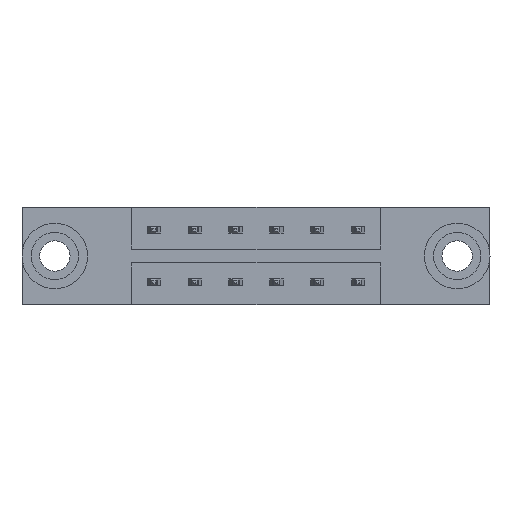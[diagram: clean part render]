
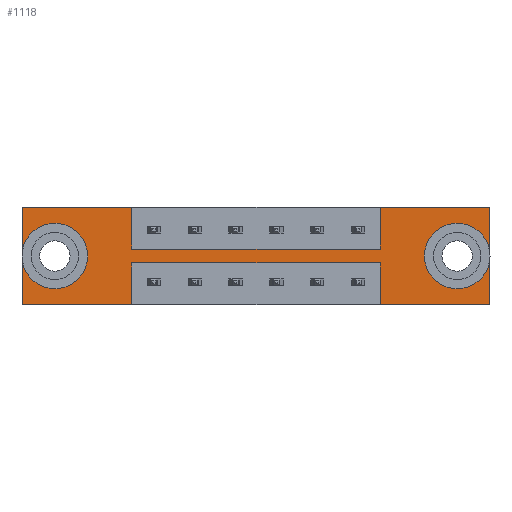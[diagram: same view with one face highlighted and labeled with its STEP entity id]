
A CAD part, front view. The second image highlights one B-rep face of the part: STEP entity #1118.
In plain terms, the highlighted planar face has unit normal (0, -1, 0).
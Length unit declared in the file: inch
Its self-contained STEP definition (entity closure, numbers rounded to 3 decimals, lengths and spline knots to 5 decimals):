
#32 = DIRECTION ( 'NONE',  ( 1., 0., 0. ) ) ;
#90 = VECTOR ( 'NONE', #867, 39.37008 ) ;
#153 = ORIENTED_EDGE ( 'NONE', *, *, #6819, .F. ) ;
#166 = CARTESIAN_POINT ( 'NONE',  ( 0., 0., 0. ) ) ;
#227 = DIRECTION ( 'NONE',  ( 0., 0., 1. ) ) ;
#283 = VERTEX_POINT ( 'NONE', #3975 ) ;
#312 = VERTEX_POINT ( 'NONE', #690 ) ;
#335 = EDGE_CURVE ( 'NONE', #312, #6142, #4841, .T. ) ;
#435 = LINE ( 'NONE', #8490, #8972 ) ;
#445 = DIRECTION ( 'NONE',  ( 0., 0., -1. ) ) ;
#528 = CARTESIAN_POINT ( 'NONE',  ( 0.4175, 0., -0.1585 ) ) ;
#538 = DIRECTION ( 'NONE',  ( 0., 0., -1. ) ) ;
#555 = EDGE_LOOP ( 'NONE', ( #7140, #1626 ) ) ;
#556 = EDGE_CURVE ( 'NONE', #1674, #4452, #4484, .T. ) ;
#621 = ORIENTED_EDGE ( 'NONE', *, *, #6482, .F. ) ;
#690 = CARTESIAN_POINT ( 'NONE',  ( 0.125, 0., -0.263 ) ) ;
#728 = CARTESIAN_POINT ( 'NONE',  ( 1.3665, 0., -0.1585 ) ) ;
#773 = CARTESIAN_POINT ( 'NONE',  ( 1.784, 0., 0. ) ) ;
#844 = ORIENTED_EDGE ( 'NONE', *, *, #7624, .F. ) ;
#867 = DIRECTION ( 'NONE',  ( 0., 0., 1. ) ) ;
#1046 = LINE ( 'NONE', #9149, #8395 ) ;
#1118 = ADVANCED_FACE ( 'NONE', ( #2104, #5496, #7355 ), #1302, .T. ) ;
#1302 = PLANE ( 'NONE',  #3380 ) ;
#1351 = VERTEX_POINT ( 'NONE', #7429 ) ;
#1425 = CARTESIAN_POINT ( 'NONE',  ( 0., 0., -0.37 ) ) ;
#1592 = LINE ( 'NONE', #8271, #6138 ) ;
#1626 = ORIENTED_EDGE ( 'NONE', *, *, #7099, .T. ) ;
#1674 = VERTEX_POINT ( 'NONE', #3363 ) ;
#1823 = CARTESIAN_POINT ( 'NONE',  ( 0.4175, 0., -0.1585 ) ) ;
#1852 = ORIENTED_EDGE ( 'NONE', *, *, #8261, .F. ) ;
#1972 = VERTEX_POINT ( 'NONE', #3911 ) ;
#2020 = DIRECTION ( 'NONE',  ( 0., 0., -1. ) ) ;
#2021 = VERTEX_POINT ( 'NONE', #8206 ) ;
#2055 = DIRECTION ( 'NONE',  ( -1., 0., 0. ) ) ;
#2104 = FACE_BOUND ( 'NONE', #555, .T. ) ;
#2151 = CARTESIAN_POINT ( 'NONE',  ( 0., 0., -0.37 ) ) ;
#2260 = DIRECTION ( 'NONE',  ( 0., -1., 0. ) ) ;
#2391 = EDGE_CURVE ( 'NONE', #6142, #312, #8800, .T. ) ;
#2453 = LINE ( 'NONE', #528, #6045 ) ;
#2458 = VERTEX_POINT ( 'NONE', #1425 ) ;
#2579 = ORIENTED_EDGE ( 'NONE', *, *, #3191, .F. ) ;
#2624 = VECTOR ( 'NONE', #5005, 39.37008 ) ;
#2634 = CARTESIAN_POINT ( 'NONE',  ( 1.659, 0., -0.263 ) ) ;
#2798 = CARTESIAN_POINT ( 'NONE',  ( 1.784, 0., -0.37 ) ) ;
#3191 = EDGE_CURVE ( 'NONE', #2458, #3700, #5799, .T. ) ;
#3336 = EDGE_CURVE ( 'NONE', #5399, #4900, #6786, .T. ) ;
#3363 = CARTESIAN_POINT ( 'NONE',  ( 1.3665, 0., 0. ) ) ;
#3380 = AXIS2_PLACEMENT_3D ( 'NONE', #2151, #2260, #2020 ) ;
#3385 = CARTESIAN_POINT ( 'NONE',  ( 0.125, 0., -0.185 ) ) ;
#3482 = EDGE_LOOP ( 'NONE', ( #1852, #7568, #153, #4021, #5942, #7802, #8017, #621, #2579, #4474, #8227, #844 ) ) ;
#3700 = VERTEX_POINT ( 'NONE', #8717 ) ;
#3808 = EDGE_CURVE ( 'NONE', #7415, #7008, #6336, .T. ) ;
#3911 = CARTESIAN_POINT ( 'NONE',  ( 0.4175, 0., -0.37 ) ) ;
#3951 = LINE ( 'NONE', #7084, #7502 ) ;
#3975 = CARTESIAN_POINT ( 'NONE',  ( 1.3665, 0., -0.2115 ) ) ;
#4021 = ORIENTED_EDGE ( 'NONE', *, *, #556, .F. ) ;
#4245 = DIRECTION ( 'NONE',  ( 0., 0., -1. ) ) ;
#4259 = DIRECTION ( 'NONE',  ( 0., 1., 0. ) ) ;
#4308 = CARTESIAN_POINT ( 'NONE',  ( 1.659, 0., -0.185 ) ) ;
#4431 = VECTOR ( 'NONE', #8244, 39.37008 ) ;
#4435 = VECTOR ( 'NONE', #445, 39.37008 ) ;
#4452 = VERTEX_POINT ( 'NONE', #5290 ) ;
#4474 = ORIENTED_EDGE ( 'NONE', *, *, #5937, .F. ) ;
#4482 = EDGE_CURVE ( 'NONE', #6966, #8374, #6436, .T. ) ;
#4484 = LINE ( 'NONE', #166, #4719 ) ;
#4719 = VECTOR ( 'NONE', #32, 39.37008 ) ;
#4841 = CIRCLE ( 'NONE', #4905, 0.078 ) ;
#4900 = VERTEX_POINT ( 'NONE', #2634 ) ;
#4905 = AXIS2_PLACEMENT_3D ( 'NONE', #3385, #5890, #6672 ) ;
#5005 = DIRECTION ( 'NONE',  ( -1., 0., 0. ) ) ;
#5064 = CARTESIAN_POINT ( 'NONE',  ( 0., 0., -0.37 ) ) ;
#5273 = EDGE_CURVE ( 'NONE', #1351, #7415, #2453, .T. ) ;
#5290 = CARTESIAN_POINT ( 'NONE',  ( 1.784, 0., 0. ) ) ;
#5399 = VERTEX_POINT ( 'NONE', #7959 ) ;
#5494 = ORIENTED_EDGE ( 'NONE', *, *, #2391, .T. ) ;
#5496 = FACE_BOUND ( 'NONE', #6860, .T. ) ;
#5787 = CIRCLE ( 'NONE', #8118, 0.078 ) ;
#5799 = LINE ( 'NONE', #6702, #9199 ) ;
#5887 = LINE ( 'NONE', #5931, #90 ) ;
#5890 = DIRECTION ( 'NONE',  ( 0., 1., 0. ) ) ;
#5931 = CARTESIAN_POINT ( 'NONE',  ( 1.3665, 0., -0.1585 ) ) ;
#5937 = EDGE_CURVE ( 'NONE', #1972, #2458, #1046, .T. ) ;
#5942 = ORIENTED_EDGE ( 'NONE', *, *, #7806, .F. ) ;
#6045 = VECTOR ( 'NONE', #538, 39.37008 ) ;
#6138 = VECTOR ( 'NONE', #8538, 39.37008 ) ;
#6142 = VERTEX_POINT ( 'NONE', #6556 ) ;
#6336 = LINE ( 'NONE', #8282, #4431 ) ;
#6343 = LINE ( 'NONE', #773, #4435 ) ;
#6362 = DIRECTION ( 'NONE',  ( 0., 0., 1. ) ) ;
#6436 = LINE ( 'NONE', #5064, #2624 ) ;
#6467 = AXIS2_PLACEMENT_3D ( 'NONE', #4308, #4259, #4245 ) ;
#6482 = EDGE_CURVE ( 'NONE', #3700, #1351, #1592, .T. ) ;
#6525 = AXIS2_PLACEMENT_3D ( 'NONE', #7811, #8815, #227 ) ;
#6556 = CARTESIAN_POINT ( 'NONE',  ( 0.125, 0., -0.107 ) ) ;
#6672 = DIRECTION ( 'NONE',  ( 0., 0., 1. ) ) ;
#6702 = CARTESIAN_POINT ( 'NONE',  ( 0., 0., 0. ) ) ;
#6786 = CIRCLE ( 'NONE', #6467, 0.078 ) ;
#6819 = EDGE_CURVE ( 'NONE', #4452, #6966, #6343, .T. ) ;
#6860 = EDGE_LOOP ( 'NONE', ( #5494, #7354 ) ) ;
#6966 = VERTEX_POINT ( 'NONE', #2798 ) ;
#6984 = VECTOR ( 'NONE', #7485, 39.37008 ) ;
#7008 = VERTEX_POINT ( 'NONE', #728 ) ;
#7084 = CARTESIAN_POINT ( 'NONE',  ( 1.3665, 0., -0.2115 ) ) ;
#7099 = EDGE_CURVE ( 'NONE', #4900, #5399, #5787, .T. ) ;
#7140 = ORIENTED_EDGE ( 'NONE', *, *, #3336, .T. ) ;
#7163 = EDGE_CURVE ( 'NONE', #2021, #1972, #9189, .T. ) ;
#7232 = CARTESIAN_POINT ( 'NONE',  ( 1.3665, 0., -0.37 ) ) ;
#7354 = ORIENTED_EDGE ( 'NONE', *, *, #335, .T. ) ;
#7355 = FACE_OUTER_BOUND ( 'NONE', #3482, .T. ) ;
#7386 = CARTESIAN_POINT ( 'NONE',  ( 0.4175, 0., -0.2115 ) ) ;
#7415 = VERTEX_POINT ( 'NONE', #1823 ) ;
#7429 = CARTESIAN_POINT ( 'NONE',  ( 0.4175, 0., 0. ) ) ;
#7485 = DIRECTION ( 'NONE',  ( 0., 0., -1. ) ) ;
#7502 = VECTOR ( 'NONE', #7787, 39.37008 ) ;
#7568 = ORIENTED_EDGE ( 'NONE', *, *, #4482, .F. ) ;
#7624 = EDGE_CURVE ( 'NONE', #283, #2021, #435, .T. ) ;
#7787 = DIRECTION ( 'NONE',  ( 0., 0., 1. ) ) ;
#7802 = ORIENTED_EDGE ( 'NONE', *, *, #3808, .F. ) ;
#7806 = EDGE_CURVE ( 'NONE', #7008, #1674, #5887, .T. ) ;
#7811 = CARTESIAN_POINT ( 'NONE',  ( 0.125, 0., -0.185 ) ) ;
#7831 = DIRECTION ( 'NONE',  ( -1., 0., 0. ) ) ;
#7959 = CARTESIAN_POINT ( 'NONE',  ( 1.659, 0., -0.107 ) ) ;
#7995 = DIRECTION ( 'NONE',  ( 0., 0., -1. ) ) ;
#8017 = ORIENTED_EDGE ( 'NONE', *, *, #5273, .F. ) ;
#8022 = DIRECTION ( 'NONE',  ( 0., 1., 0. ) ) ;
#8048 = CARTESIAN_POINT ( 'NONE',  ( 1.659, 0., -0.185 ) ) ;
#8118 = AXIS2_PLACEMENT_3D ( 'NONE', #8048, #8022, #7995 ) ;
#8206 = CARTESIAN_POINT ( 'NONE',  ( 0.4175, 0., -0.2115 ) ) ;
#8227 = ORIENTED_EDGE ( 'NONE', *, *, #7163, .F. ) ;
#8244 = DIRECTION ( 'NONE',  ( 1., 0., 0. ) ) ;
#8261 = EDGE_CURVE ( 'NONE', #8374, #283, #3951, .T. ) ;
#8271 = CARTESIAN_POINT ( 'NONE',  ( 0., 0., 0. ) ) ;
#8282 = CARTESIAN_POINT ( 'NONE',  ( 0.4175, 0., -0.1585 ) ) ;
#8374 = VERTEX_POINT ( 'NONE', #7232 ) ;
#8395 = VECTOR ( 'NONE', #2055, 39.37008 ) ;
#8490 = CARTESIAN_POINT ( 'NONE',  ( 0.4175, 0., -0.2115 ) ) ;
#8538 = DIRECTION ( 'NONE',  ( 1., 0., 0. ) ) ;
#8717 = CARTESIAN_POINT ( 'NONE',  ( 0., 0., 0. ) ) ;
#8800 = CIRCLE ( 'NONE', #6525, 0.078 ) ;
#8815 = DIRECTION ( 'NONE',  ( 0., 1., 0. ) ) ;
#8972 = VECTOR ( 'NONE', #7831, 39.37008 ) ;
#9149 = CARTESIAN_POINT ( 'NONE',  ( 0., 0., -0.37 ) ) ;
#9189 = LINE ( 'NONE', #7386, #6984 ) ;
#9199 = VECTOR ( 'NONE', #6362, 39.37008 ) ;
